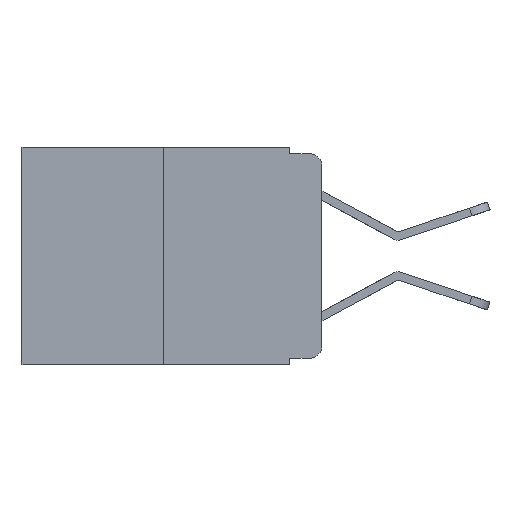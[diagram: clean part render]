
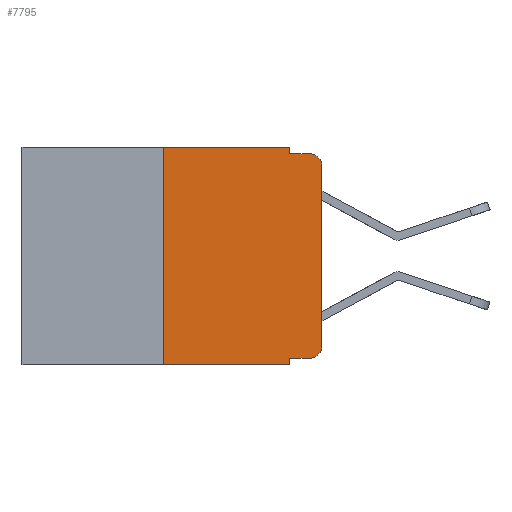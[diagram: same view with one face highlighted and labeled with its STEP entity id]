
A CAD part, left-side view. The second image highlights one B-rep face of the part: STEP entity #7795.
In plain terms, the highlighted planar face has unit normal (-1, 0, 0).
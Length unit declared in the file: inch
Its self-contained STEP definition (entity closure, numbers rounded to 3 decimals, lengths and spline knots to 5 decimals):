
#93 = DIRECTION ( 'NONE',  ( 0., 0., 1. ) ) ;
#108 = CIRCLE ( 'NONE', #2877, 0.02 ) ;
#207 = CARTESIAN_POINT ( 'NONE',  ( 0., 0.02, -0.01 ) ) ;
#336 = CARTESIAN_POINT ( 'NONE',  ( 0., 0., 0. ) ) ;
#388 = VECTOR ( 'NONE', #93, 39.37008 ) ;
#434 = CARTESIAN_POINT ( 'NONE',  ( 0., 0., -0.313 ) ) ;
#453 = DIRECTION ( 'NONE',  ( 0., 0., -1. ) ) ;
#533 = FACE_OUTER_BOUND ( 'NONE', #4283, .T. ) ;
#585 = CARTESIAN_POINT ( 'NONE',  ( 0., 0.051, 0. ) ) ;
#814 = VERTEX_POINT ( 'NONE', #10259 ) ;
#1233 = LINE ( 'NONE', #3720, #5894 ) ;
#1606 = CARTESIAN_POINT ( 'NONE',  ( 0., 0., -0.03 ) ) ;
#1865 = VECTOR ( 'NONE', #10657, 39.37008 ) ;
#2003 = VECTOR ( 'NONE', #7323, 39.37008 ) ;
#2047 = EDGE_CURVE ( 'NONE', #8501, #8622, #7520, .T. ) ;
#2110 = CARTESIAN_POINT ( 'NONE',  ( 0., 0.02, -0.03 ) ) ;
#2499 = ORIENTED_EDGE ( 'NONE', *, *, #6987, .F. ) ;
#2700 = CARTESIAN_POINT ( 'NONE',  ( 0., 0.473, 0. ) ) ;
#2877 = AXIS2_PLACEMENT_3D ( 'NONE', #2954, #9150, #3882 ) ;
#2954 = CARTESIAN_POINT ( 'NONE',  ( 0., 0.02, -0.313 ) ) ;
#2965 = AXIS2_PLACEMENT_3D ( 'NONE', #4290, #6114, #453 ) ;
#3058 = DIRECTION ( 'NONE',  ( 0., 0., -1. ) ) ;
#3294 = VERTEX_POINT ( 'NONE', #207 ) ;
#3676 = ORIENTED_EDGE ( 'NONE', *, *, #5799, .T. ) ;
#3691 = VERTEX_POINT ( 'NONE', #10994 ) ;
#3720 = CARTESIAN_POINT ( 'NONE',  ( 0., 0.051, -0.333 ) ) ;
#3882 = DIRECTION ( 'NONE',  ( 0., 0., -1. ) ) ;
#3988 = VECTOR ( 'NONE', #8070, 39.37008 ) ;
#4153 = LINE ( 'NONE', #9736, #8831 ) ;
#4227 = CIRCLE ( 'NONE', #5762, 0.02 ) ;
#4283 = EDGE_LOOP ( 'NONE', ( #11550, #11383, #11191, #11181, #7602, #5529, #10758, #2499, #5496, #3676 ) ) ;
#4290 = CARTESIAN_POINT ( 'NONE',  ( 0., 0.473, 0. ) ) ;
#4340 = LINE ( 'NONE', #2700, #1865 ) ;
#4394 = DIRECTION ( 'NONE',  ( 0., -1., 0. ) ) ;
#4447 = LINE ( 'NONE', #5553, #2003 ) ;
#4872 = CARTESIAN_POINT ( 'NONE',  ( 0., 0.25, 0. ) ) ;
#5270 = EDGE_CURVE ( 'NONE', #8622, #3294, #4227, .T. ) ;
#5353 = DIRECTION ( 'NONE',  ( 0., -1., 0. ) ) ;
#5408 = CARTESIAN_POINT ( 'NONE',  ( 0., 0.051, 0. ) ) ;
#5423 = CARTESIAN_POINT ( 'NONE',  ( 0., 0.051, -0.343 ) ) ;
#5496 = ORIENTED_EDGE ( 'NONE', *, *, #6395, .T. ) ;
#5529 = ORIENTED_EDGE ( 'NONE', *, *, #7563, .F. ) ;
#5540 = VECTOR ( 'NONE', #4394, 39.37008 ) ;
#5553 = CARTESIAN_POINT ( 'NONE',  ( 0., 0.051, 0. ) ) ;
#5762 = AXIS2_PLACEMENT_3D ( 'NONE', #2110, #8383, #3058 ) ;
#5799 = EDGE_CURVE ( 'NONE', #7051, #8501, #108, .T. ) ;
#5894 = VECTOR ( 'NONE', #6459, 39.37008 ) ;
#6021 = LINE ( 'NONE', #4872, #388 ) ;
#6114 = DIRECTION ( 'NONE',  ( 1., 0., 0. ) ) ;
#6328 = EDGE_CURVE ( 'NONE', #10517, #11540, #4340, .T. ) ;
#6395 = EDGE_CURVE ( 'NONE', #11402, #7051, #1233, .T. ) ;
#6459 = DIRECTION ( 'NONE',  ( 0., -1., 0. ) ) ;
#6987 = EDGE_CURVE ( 'NONE', #11402, #8020, #4447, .T. ) ;
#7051 = VERTEX_POINT ( 'NONE', #11629 ) ;
#7323 = DIRECTION ( 'NONE',  ( 0., 0., -1. ) ) ;
#7520 = LINE ( 'NONE', #336, #9545 ) ;
#7563 = EDGE_CURVE ( 'NONE', #3691, #10517, #6021, .T. ) ;
#7602 = ORIENTED_EDGE ( 'NONE', *, *, #6328, .F. ) ;
#7795 = ADVANCED_FACE ( 'NONE', ( #533 ), #7828, .F. ) ;
#7828 = PLANE ( 'NONE',  #2965 ) ;
#7952 = EDGE_CURVE ( 'NONE', #3691, #8020, #4153, .T. ) ;
#8020 = VERTEX_POINT ( 'NONE', #5423 ) ;
#8070 = DIRECTION ( 'NONE',  ( 0., 0., -1. ) ) ;
#8383 = DIRECTION ( 'NONE',  ( -1., 0., 0. ) ) ;
#8501 = VERTEX_POINT ( 'NONE', #434 ) ;
#8622 = VERTEX_POINT ( 'NONE', #1606 ) ;
#8656 = CARTESIAN_POINT ( 'NONE',  ( 0., 0.051, -0.333 ) ) ;
#8696 = LINE ( 'NONE', #5408, #3988 ) ;
#8717 = EDGE_CURVE ( 'NONE', #11540, #814, #8696, .T. ) ;
#8831 = VECTOR ( 'NONE', #5353, 39.37008 ) ;
#9150 = DIRECTION ( 'NONE',  ( -1., 0., 0. ) ) ;
#9545 = VECTOR ( 'NONE', #11430, 39.37008 ) ;
#9664 = CARTESIAN_POINT ( 'NONE',  ( 0., 0.051, -0.01 ) ) ;
#9736 = CARTESIAN_POINT ( 'NONE',  ( 0., 0.473, -0.343 ) ) ;
#9869 = EDGE_CURVE ( 'NONE', #814, #3294, #10170, .T. ) ;
#10170 = LINE ( 'NONE', #9664, #5540 ) ;
#10259 = CARTESIAN_POINT ( 'NONE',  ( 0., 0.051, -0.01 ) ) ;
#10517 = VERTEX_POINT ( 'NONE', #11428 ) ;
#10657 = DIRECTION ( 'NONE',  ( 0., -1., 0. ) ) ;
#10758 = ORIENTED_EDGE ( 'NONE', *, *, #7952, .T. ) ;
#10994 = CARTESIAN_POINT ( 'NONE',  ( 0., 0.25, -0.343 ) ) ;
#11181 = ORIENTED_EDGE ( 'NONE', *, *, #8717, .F. ) ;
#11191 = ORIENTED_EDGE ( 'NONE', *, *, #9869, .F. ) ;
#11383 = ORIENTED_EDGE ( 'NONE', *, *, #5270, .T. ) ;
#11402 = VERTEX_POINT ( 'NONE', #8656 ) ;
#11428 = CARTESIAN_POINT ( 'NONE',  ( 0., 0.25, 0. ) ) ;
#11430 = DIRECTION ( 'NONE',  ( 0., 0., 1. ) ) ;
#11540 = VERTEX_POINT ( 'NONE', #585 ) ;
#11550 = ORIENTED_EDGE ( 'NONE', *, *, #2047, .T. ) ;
#11629 = CARTESIAN_POINT ( 'NONE',  ( 0., 0.02, -0.333 ) ) ;
